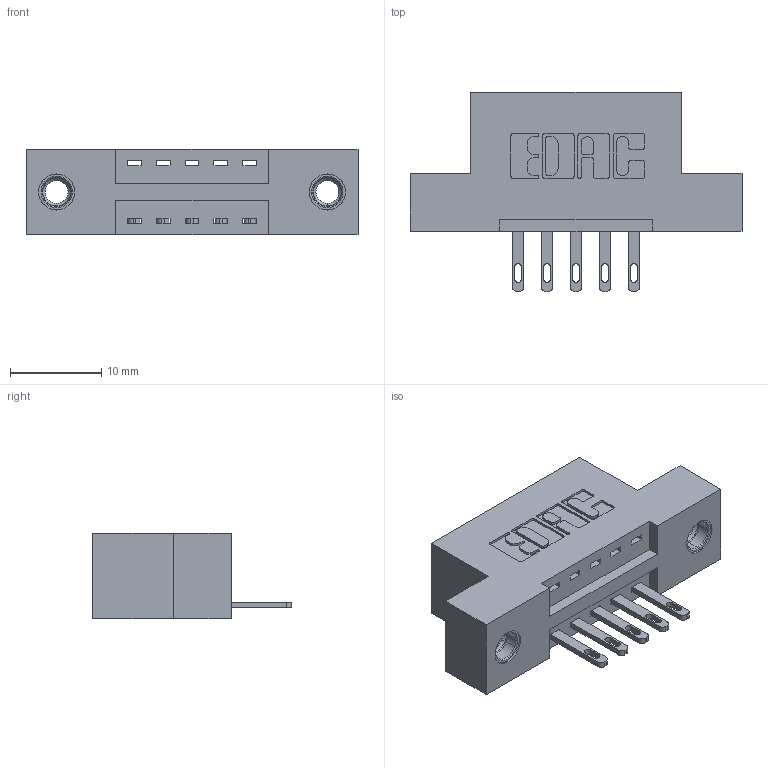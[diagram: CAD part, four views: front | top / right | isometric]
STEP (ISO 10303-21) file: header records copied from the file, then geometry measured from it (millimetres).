
FILE_DESCRIPTION (( 'STEP AP203' ), '1' );
FILE_NAME ('346-005-500-107.STEP', '2022-05-04T17:18:51', ( '' ), ( '' ), 'SwSTEP 2.0', 'SolidWorks 2020', '' );
FILE_SCHEMA (( 'CONFIG_CONTROL_DESIGN' ));
Length unit declared in the file: inch
Products named in the file (4): 345-292-001_345-293-100; 346-005-500-107; 346 Part_Flush Mounting Lugs - 0.156 Dia-TI; 345-250-001_345-250-005-103
Assembly tree (8 placements, depth 2):
  346-005-500-107
    346 Part_Flush Mounting Lugs - 0.156 Dia-TI
    345-292-001_345-293-100  x5
    345-250-001_345-250-005-103  x2
Bounding box: 36.45 x 21.84 x 9.4 mm (x, y, z)
Volume: 3223.6 mm3; surface area: 3676.1 mm2
Topology: 8 solids, 8 shells, 452 faces, 1305 edges, 862 vertices
Faces by surface type: plane 278, cylinder 158, cone 12, torus 4
Entity records: 9200 total; most frequent: CARTESIAN_POINT 1570, ORIENTED_EDGE 1502, DIRECTION 1459, EDGE_CURVE 751, LINE 575, VECTOR 575, VERTEX_POINT 496, AXIS2_PLACEMENT_3D 442
